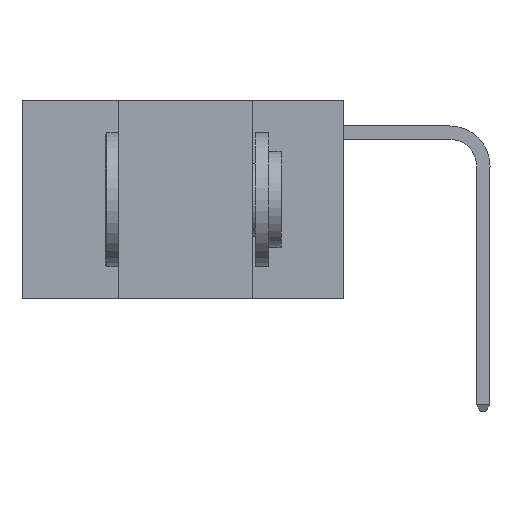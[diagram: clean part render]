
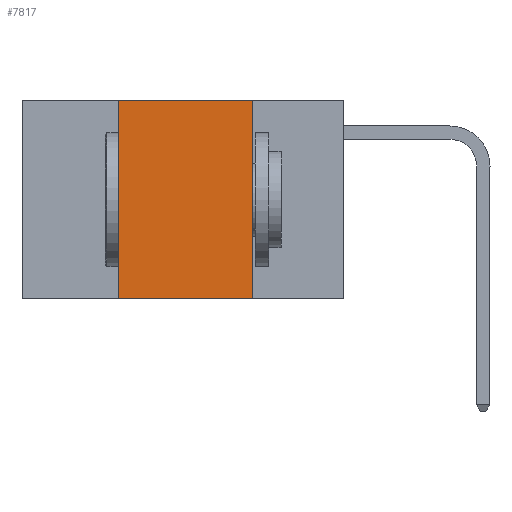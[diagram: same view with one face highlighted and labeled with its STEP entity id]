
A CAD part, left-side view. The second image highlights one B-rep face of the part: STEP entity #7817.
In plain terms, the highlighted planar face has unit normal (-1, 0, 0).
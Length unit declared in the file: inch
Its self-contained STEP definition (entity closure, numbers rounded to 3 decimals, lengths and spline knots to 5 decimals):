
#477 = CARTESIAN_POINT ( 'NONE',  ( 0., 0.6, -0.37 ) ) ;
#1336 = ORIENTED_EDGE ( 'NONE', *, *, #13897, .F. ) ;
#1975 = EDGE_LOOP ( 'NONE', ( #9968, #1336, #4376, #7392 ) ) ;
#2460 = DIRECTION ( 'NONE',  ( 0., 0., 1. ) ) ;
#2665 = LINE ( 'NONE', #11397, #6001 ) ;
#2936 = LINE ( 'NONE', #3625, #14096 ) ;
#3233 = LINE ( 'NONE', #477, #8840 ) ;
#3584 = PLANE ( 'NONE',  #13038 ) ;
#3625 = CARTESIAN_POINT ( 'NONE',  ( 0., 0.42, 0. ) ) ;
#4126 = LINE ( 'NONE', #11459, #6761 ) ;
#4376 = ORIENTED_EDGE ( 'NONE', *, *, #11404, .F. ) ;
#4712 = VERTEX_POINT ( 'NONE', #5414 ) ;
#4743 = DIRECTION ( 'NONE',  ( 0., 0., -1. ) ) ;
#5414 = CARTESIAN_POINT ( 'NONE',  ( 0., 0.42, -0.37 ) ) ;
#6001 = VECTOR ( 'NONE', #12417, 39.37008 ) ;
#6292 = VERTEX_POINT ( 'NONE', #6301 ) ;
#6301 = CARTESIAN_POINT ( 'NONE',  ( 0., 0.17, 0. ) ) ;
#6761 = VECTOR ( 'NONE', #12472, 39.37008 ) ;
#7392 = ORIENTED_EDGE ( 'NONE', *, *, #7447, .T. ) ;
#7447 = EDGE_CURVE ( 'NONE', #4712, #9035, #3233, .T. ) ;
#7542 = CARTESIAN_POINT ( 'NONE',  ( 0., 0.17, -0.37 ) ) ;
#7817 = ADVANCED_FACE ( 'NONE', ( #9840 ), #3584, .F. ) ;
#8143 = CARTESIAN_POINT ( 'NONE',  ( 0., 0.42, 0. ) ) ;
#8724 = VERTEX_POINT ( 'NONE', #8143 ) ;
#8759 = EDGE_CURVE ( 'NONE', #6292, #9035, #2665, .T. ) ;
#8840 = VECTOR ( 'NONE', #11705, 39.37008 ) ;
#9035 = VERTEX_POINT ( 'NONE', #7542 ) ;
#9840 = FACE_OUTER_BOUND ( 'NONE', #1975, .T. ) ;
#9968 = ORIENTED_EDGE ( 'NONE', *, *, #8759, .F. ) ;
#11295 = CARTESIAN_POINT ( 'NONE',  ( 0., 0.6, 0. ) ) ;
#11340 = DIRECTION ( 'NONE',  ( 1., 0., 0. ) ) ;
#11397 = CARTESIAN_POINT ( 'NONE',  ( 0., 0.17, 0. ) ) ;
#11404 = EDGE_CURVE ( 'NONE', #4712, #8724, #2936, .T. ) ;
#11459 = CARTESIAN_POINT ( 'NONE',  ( 0., 0.6, 0. ) ) ;
#11705 = DIRECTION ( 'NONE',  ( 0., -1., 0. ) ) ;
#12417 = DIRECTION ( 'NONE',  ( 0., 0., -1. ) ) ;
#12472 = DIRECTION ( 'NONE',  ( 0., -1., 0. ) ) ;
#13038 = AXIS2_PLACEMENT_3D ( 'NONE', #11295, #11340, #4743 ) ;
#13897 = EDGE_CURVE ( 'NONE', #8724, #6292, #4126, .T. ) ;
#14096 = VECTOR ( 'NONE', #2460, 39.37008 ) ;
